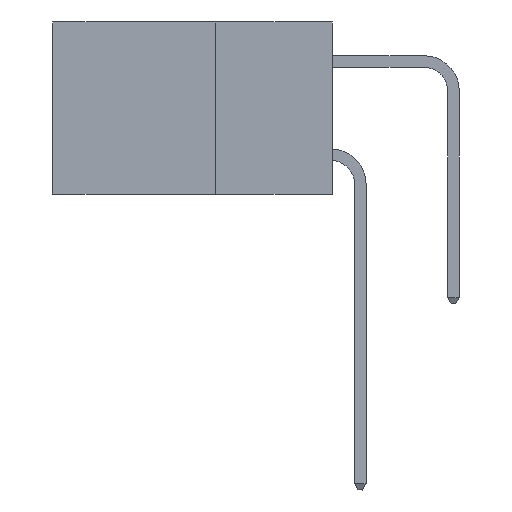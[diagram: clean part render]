
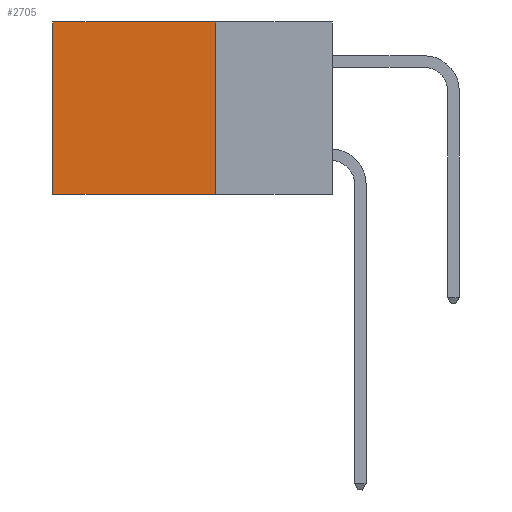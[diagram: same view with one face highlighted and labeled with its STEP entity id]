
A CAD part, left-side view. The second image highlights one B-rep face of the part: STEP entity #2705.
In plain terms, the highlighted planar face has unit normal (-1, 0, 0).
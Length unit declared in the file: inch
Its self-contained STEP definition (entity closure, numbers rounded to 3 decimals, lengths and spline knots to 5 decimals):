
#117 = ORIENTED_EDGE ( 'NONE', *, *, #8640, .T. ) ;
#311 = EDGE_CURVE ( 'NONE', #4126, #6757, #10414, .T. ) ;
#356 = FACE_OUTER_BOUND ( 'NONE', #6549, .T. ) ;
#1061 = CARTESIAN_POINT ( 'NONE',  ( 0.298, 0.6, 0. ) ) ;
#2067 = DIRECTION ( 'NONE',  ( 0., 0., -1. ) ) ;
#2383 = ORIENTED_EDGE ( 'NONE', *, *, #311, .F. ) ;
#2705 = ADVANCED_FACE ( 'NONE', ( #356 ), #7723, .F. ) ;
#3570 = EDGE_CURVE ( 'NONE', #4126, #4978, #13187, .T. ) ;
#4126 = VERTEX_POINT ( 'NONE', #10191 ) ;
#4978 = VERTEX_POINT ( 'NONE', #1061 ) ;
#4984 = EDGE_CURVE ( 'NONE', #6757, #8348, #6827, .T. ) ;
#5316 = AXIS2_PLACEMENT_3D ( 'NONE', #10126, #13604, #8829 ) ;
#5635 = CARTESIAN_POINT ( 'NONE',  ( 0.298, 0.25, 0. ) ) ;
#6549 = EDGE_LOOP ( 'NONE', ( #117, #10908, #2383, #11171 ) ) ;
#6757 = VERTEX_POINT ( 'NONE', #9244 ) ;
#6827 = LINE ( 'NONE', #6896, #8980 ) ;
#6896 = CARTESIAN_POINT ( 'NONE',  ( 0.298, 0.25, -0.37 ) ) ;
#7381 = VECTOR ( 'NONE', #13144, 39.37008 ) ;
#7723 = PLANE ( 'NONE',  #5316 ) ;
#8035 = VECTOR ( 'NONE', #2067, 39.37008 ) ;
#8348 = VERTEX_POINT ( 'NONE', #10309 ) ;
#8640 = EDGE_CURVE ( 'NONE', #4978, #8348, #9494, .T. ) ;
#8829 = DIRECTION ( 'NONE',  ( 0., 0., -1. ) ) ;
#8980 = VECTOR ( 'NONE', #14985, 39.37008 ) ;
#9244 = CARTESIAN_POINT ( 'NONE',  ( 0.298, 0.25, -0.37 ) ) ;
#9286 = CARTESIAN_POINT ( 'NONE',  ( 0.298, 0.6, 0. ) ) ;
#9494 = LINE ( 'NONE', #9286, #11860 ) ;
#10126 = CARTESIAN_POINT ( 'NONE',  ( 0.298, 0.25, 0. ) ) ;
#10191 = CARTESIAN_POINT ( 'NONE',  ( 0.298, 0.25, 0. ) ) ;
#10309 = CARTESIAN_POINT ( 'NONE',  ( 0.298, 0.6, -0.37 ) ) ;
#10414 = LINE ( 'NONE', #5635, #8035 ) ;
#10908 = ORIENTED_EDGE ( 'NONE', *, *, #4984, .F. ) ;
#11171 = ORIENTED_EDGE ( 'NONE', *, *, #3570, .T. ) ;
#11860 = VECTOR ( 'NONE', #14056, 39.37008 ) ;
#13144 = DIRECTION ( 'NONE',  ( 0., 1., 0. ) ) ;
#13187 = LINE ( 'NONE', #14291, #7381 ) ;
#13604 = DIRECTION ( 'NONE',  ( 1., 0., 0. ) ) ;
#14056 = DIRECTION ( 'NONE',  ( 0., 0., -1. ) ) ;
#14291 = CARTESIAN_POINT ( 'NONE',  ( 0.298, 0.25, 0. ) ) ;
#14985 = DIRECTION ( 'NONE',  ( 0., 1., 0. ) ) ;
